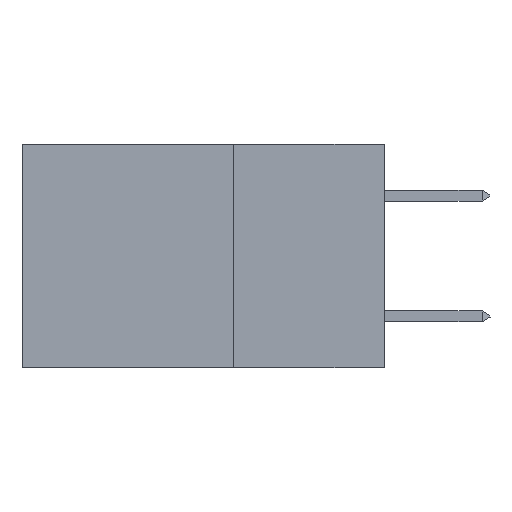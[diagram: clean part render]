
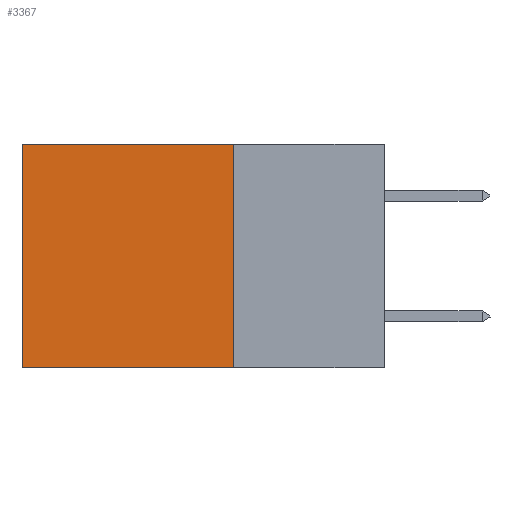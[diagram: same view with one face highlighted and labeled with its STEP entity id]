
A CAD part, left-side view. The second image highlights one B-rep face of the part: STEP entity #3367.
In plain terms, the highlighted planar face has unit normal (-1, 0, 0).
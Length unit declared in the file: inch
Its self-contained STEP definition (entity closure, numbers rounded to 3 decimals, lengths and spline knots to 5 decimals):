
#190 = LINE ( 'NONE', #16141, #2598 ) ;
#602 = AXIS2_PLACEMENT_3D ( 'NONE', #12957, #2626, #16706 ) ;
#1474 = EDGE_CURVE ( 'NONE', #7208, #2117, #190, .T. ) ;
#1609 = FACE_OUTER_BOUND ( 'NONE', #3280, .T. ) ;
#2117 = VERTEX_POINT ( 'NONE', #8107 ) ;
#2360 = CARTESIAN_POINT ( 'NONE',  ( 0.2875, 0.25, 0. ) ) ;
#2577 = PLANE ( 'NONE',  #602 ) ;
#2598 = VECTOR ( 'NONE', #11126, 39.37008 ) ;
#2626 = DIRECTION ( 'NONE',  ( 1., 0., 0. ) ) ;
#2738 = EDGE_CURVE ( 'NONE', #7208, #12523, #12060, .T. ) ;
#3152 = EDGE_CURVE ( 'NONE', #2117, #9398, #14051, .T. ) ;
#3280 = EDGE_LOOP ( 'NONE', ( #4636, #10149, #8305, #15708 ) ) ;
#3367 = ADVANCED_FACE ( 'NONE', ( #1609 ), #2577, .F. ) ;
#4636 = ORIENTED_EDGE ( 'NONE', *, *, #3152, .T. ) ;
#4868 = VECTOR ( 'NONE', #11511, 39.37008 ) ;
#5053 = CARTESIAN_POINT ( 'NONE',  ( 0.2875, 0.25, -0.37 ) ) ;
#5875 = CARTESIAN_POINT ( 'NONE',  ( 0.2875, 0.6, 0. ) ) ;
#6934 = CARTESIAN_POINT ( 'NONE',  ( 0.2875, 0.6, -0.37 ) ) ;
#7208 = VERTEX_POINT ( 'NONE', #15932 ) ;
#8069 = EDGE_CURVE ( 'NONE', #12523, #9398, #14916, .T. ) ;
#8107 = CARTESIAN_POINT ( 'NONE',  ( 0.2875, 0.6, 0. ) ) ;
#8305 = ORIENTED_EDGE ( 'NONE', *, *, #2738, .F. ) ;
#9398 = VERTEX_POINT ( 'NONE', #6934 ) ;
#9700 = DIRECTION ( 'NONE',  ( 0., 0., -1. ) ) ;
#10149 = ORIENTED_EDGE ( 'NONE', *, *, #8069, .F. ) ;
#10346 = CARTESIAN_POINT ( 'NONE',  ( 0.2875, 0.25, -0.37 ) ) ;
#11126 = DIRECTION ( 'NONE',  ( 0., 1., 0. ) ) ;
#11511 = DIRECTION ( 'NONE',  ( 0., 0., -1. ) ) ;
#12060 = LINE ( 'NONE', #2360, #4868 ) ;
#12523 = VERTEX_POINT ( 'NONE', #10346 ) ;
#12957 = CARTESIAN_POINT ( 'NONE',  ( 0.2875, 0.25, 0. ) ) ;
#14051 = LINE ( 'NONE', #5875, #16502 ) ;
#14916 = LINE ( 'NONE', #5053, #16731 ) ;
#15708 = ORIENTED_EDGE ( 'NONE', *, *, #1474, .T. ) ;
#15932 = CARTESIAN_POINT ( 'NONE',  ( 0.2875, 0.25, 0. ) ) ;
#16141 = CARTESIAN_POINT ( 'NONE',  ( 0.2875, 0.25, 0. ) ) ;
#16502 = VECTOR ( 'NONE', #9700, 39.37008 ) ;
#16706 = DIRECTION ( 'NONE',  ( 0., 0., -1. ) ) ;
#16731 = VECTOR ( 'NONE', #16814, 39.37008 ) ;
#16814 = DIRECTION ( 'NONE',  ( 0., 1., 0. ) ) ;
